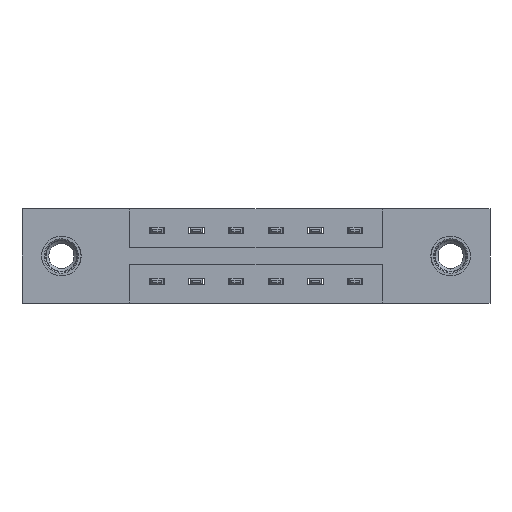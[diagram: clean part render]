
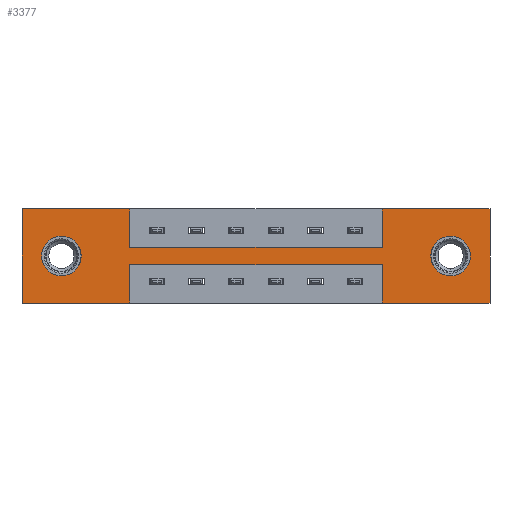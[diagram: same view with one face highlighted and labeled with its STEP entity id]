
A CAD part, front view. The second image highlights one B-rep face of the part: STEP entity #3377.
In plain terms, the highlighted planar face has unit normal (0, -1, 0).
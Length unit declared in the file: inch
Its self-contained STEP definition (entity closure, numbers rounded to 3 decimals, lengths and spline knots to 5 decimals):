
#58 = VECTOR ( 'NONE', #6489, 39.37008 ) ;
#78 = CARTESIAN_POINT ( 'NONE',  ( 0.425, 0., -0.22 ) ) ;
#393 = DIRECTION ( 'NONE',  ( 0., 1., 0. ) ) ;
#532 = DIRECTION ( 'NONE',  ( 0., 1., 0. ) ) ;
#810 = CARTESIAN_POINT ( 'NONE',  ( 0., 0., 0. ) ) ;
#1068 = DIRECTION ( 'NONE',  ( 0., 0., 1. ) ) ;
#1074 = DIRECTION ( 'NONE',  ( 0., 0., -1. ) ) ;
#1095 = CARTESIAN_POINT ( 'NONE',  ( 1.417, 0., -0.22 ) ) ;
#1121 = CARTESIAN_POINT ( 'NONE',  ( 1.687, 0., -0.263 ) ) ;
#1291 = ORIENTED_EDGE ( 'NONE', *, *, #8147, .F. ) ;
#1382 = ORIENTED_EDGE ( 'NONE', *, *, #4457, .F. ) ;
#1411 = EDGE_CURVE ( 'NONE', #7529, #3625, #1847, .T. ) ;
#1567 = EDGE_CURVE ( 'NONE', #8333, #8713, #4419, .T. ) ;
#1618 = DIRECTION ( 'NONE',  ( 0., 0., -1. ) ) ;
#1696 = EDGE_CURVE ( 'NONE', #7104, #2789, #3176, .T. ) ;
#1847 = LINE ( 'NONE', #6892, #4551 ) ;
#1904 = VECTOR ( 'NONE', #4253, 39.37008 ) ;
#2055 = CARTESIAN_POINT ( 'NONE',  ( 0.155, 0., -0.263 ) ) ;
#2165 = CARTESIAN_POINT ( 'NONE',  ( 1.842, 0., -0.37 ) ) ;
#2282 = CARTESIAN_POINT ( 'NONE',  ( 1.687, 0., -0.185 ) ) ;
#2416 = CARTESIAN_POINT ( 'NONE',  ( 0., 0., -0.37 ) ) ;
#2427 = LINE ( 'NONE', #2623, #8383 ) ;
#2592 = ORIENTED_EDGE ( 'NONE', *, *, #1411, .F. ) ;
#2623 = CARTESIAN_POINT ( 'NONE',  ( 1.842, 0., 0. ) ) ;
#2789 = VERTEX_POINT ( 'NONE', #9061 ) ;
#2800 = VERTEX_POINT ( 'NONE', #1121 ) ;
#2916 = DIRECTION ( 'NONE',  ( -1., 0., 0. ) ) ;
#3021 = EDGE_CURVE ( 'NONE', #3831, #3119, #7869, .T. ) ;
#3058 = AXIS2_PLACEMENT_3D ( 'NONE', #2416, #3770, #9369 ) ;
#3119 = VERTEX_POINT ( 'NONE', #6330 ) ;
#3174 = EDGE_CURVE ( 'NONE', #9122, #5603, #5626, .T. ) ;
#3176 = LINE ( 'NONE', #6428, #3908 ) ;
#3185 = AXIS2_PLACEMENT_3D ( 'NONE', #6871, #8557, #6077 ) ;
#3377 = ADVANCED_FACE ( 'NONE', ( #4749, #8250, #4385 ), #7163, .T. ) ;
#3480 = CARTESIAN_POINT ( 'NONE',  ( 1.417, 0., -0.37 ) ) ;
#3487 = CARTESIAN_POINT ( 'NONE',  ( 0.155, 0., -0.185 ) ) ;
#3557 = EDGE_CURVE ( 'NONE', #2800, #4116, #9262, .T. ) ;
#3574 = DIRECTION ( 'NONE',  ( 0., 0., 1. ) ) ;
#3625 = VERTEX_POINT ( 'NONE', #9545 ) ;
#3668 = DIRECTION ( 'NONE',  ( -1., 0., 0. ) ) ;
#3695 = CARTESIAN_POINT ( 'NONE',  ( 1.842, 0., 0. ) ) ;
#3770 = DIRECTION ( 'NONE',  ( 0., -1., 0. ) ) ;
#3831 = VERTEX_POINT ( 'NONE', #1095 ) ;
#3908 = VECTOR ( 'NONE', #9415, 39.37008 ) ;
#3991 = CARTESIAN_POINT ( 'NONE',  ( 0., 0., -0.37 ) ) ;
#4017 = CIRCLE ( 'NONE', #8345, 0.078 ) ;
#4115 = ORIENTED_EDGE ( 'NONE', *, *, #9272, .F. ) ;
#4116 = VERTEX_POINT ( 'NONE', #7068 ) ;
#4253 = DIRECTION ( 'NONE',  ( 1., 0., 0. ) ) ;
#4340 = LINE ( 'NONE', #9458, #9349 ) ;
#4358 = ORIENTED_EDGE ( 'NONE', *, *, #7783, .F. ) ;
#4385 = FACE_OUTER_BOUND ( 'NONE', #5245, .T. ) ;
#4419 = LINE ( 'NONE', #6917, #5160 ) ;
#4457 = EDGE_CURVE ( 'NONE', #6769, #7104, #4495, .T. ) ;
#4495 = LINE ( 'NONE', #5084, #1904 ) ;
#4551 = VECTOR ( 'NONE', #2916, 39.37008 ) ;
#4749 = FACE_BOUND ( 'NONE', #7474, .T. ) ;
#4874 = ORIENTED_EDGE ( 'NONE', *, *, #1696, .F. ) ;
#4905 = CARTESIAN_POINT ( 'NONE',  ( 0.425, 0., 0. ) ) ;
#4953 = ORIENTED_EDGE ( 'NONE', *, *, #7048, .F. ) ;
#4968 = CARTESIAN_POINT ( 'NONE',  ( 1.417, 0., -0.15 ) ) ;
#5084 = CARTESIAN_POINT ( 'NONE',  ( 0., 0., 0. ) ) ;
#5139 = ORIENTED_EDGE ( 'NONE', *, *, #9053, .T. ) ;
#5140 = ORIENTED_EDGE ( 'NONE', *, *, #3557, .T. ) ;
#5145 = LINE ( 'NONE', #810, #9289 ) ;
#5160 = VECTOR ( 'NONE', #5338, 39.37008 ) ;
#5245 = EDGE_LOOP ( 'NONE', ( #4953, #9064, #4358, #2592, #5509, #4115, #5807, #10116, #4874, #1382, #1291, #8521 ) ) ;
#5338 = DIRECTION ( 'NONE',  ( 0., 0., 1. ) ) ;
#5350 = EDGE_CURVE ( 'NONE', #2789, #8333, #4340, .T. ) ;
#5509 = ORIENTED_EDGE ( 'NONE', *, *, #9111, .F. ) ;
#5603 = VERTEX_POINT ( 'NONE', #6574 ) ;
#5626 = LINE ( 'NONE', #3991, #9633 ) ;
#5657 = CARTESIAN_POINT ( 'NONE',  ( 0., 0., 0. ) ) ;
#5807 = ORIENTED_EDGE ( 'NONE', *, *, #1567, .F. ) ;
#5898 = DIRECTION ( 'NONE',  ( 0., 0., 1. ) ) ;
#6077 = DIRECTION ( 'NONE',  ( 0., 0., -1. ) ) ;
#6239 = CARTESIAN_POINT ( 'NONE',  ( 0.425, 0., -0.37 ) ) ;
#6330 = CARTESIAN_POINT ( 'NONE',  ( 0.425, 0., -0.22 ) ) ;
#6336 = DIRECTION ( 'NONE',  ( 0., 0., 1. ) ) ;
#6371 = VECTOR ( 'NONE', #3668, 39.37008 ) ;
#6428 = CARTESIAN_POINT ( 'NONE',  ( 0.425, 0., 0. ) ) ;
#6489 = DIRECTION ( 'NONE',  ( 1., 0., 0. ) ) ;
#6550 = LINE ( 'NONE', #6862, #8673 ) ;
#6574 = CARTESIAN_POINT ( 'NONE',  ( 0., 0., -0.37 ) ) ;
#6769 = VERTEX_POINT ( 'NONE', #5657 ) ;
#6771 = LINE ( 'NONE', #3480, #8656 ) ;
#6862 = CARTESIAN_POINT ( 'NONE',  ( 0.425, 0., -0.37 ) ) ;
#6871 = CARTESIAN_POINT ( 'NONE',  ( 1.687, 0., -0.185 ) ) ;
#6892 = CARTESIAN_POINT ( 'NONE',  ( 0., 0., -0.37 ) ) ;
#6917 = CARTESIAN_POINT ( 'NONE',  ( 1.417, 0., 0. ) ) ;
#6945 = AXIS2_PLACEMENT_3D ( 'NONE', #3487, #393, #5898 ) ;
#7014 = VERTEX_POINT ( 'NONE', #2055 ) ;
#7048 = EDGE_CURVE ( 'NONE', #3119, #9122, #6550, .T. ) ;
#7068 = CARTESIAN_POINT ( 'NONE',  ( 1.687, 0., -0.107 ) ) ;
#7104 = VERTEX_POINT ( 'NONE', #4905 ) ;
#7163 = PLANE ( 'NONE',  #3058 ) ;
#7369 = CARTESIAN_POINT ( 'NONE',  ( 0., 0., 0. ) ) ;
#7474 = EDGE_LOOP ( 'NONE', ( #5139, #5140 ) ) ;
#7529 = VERTEX_POINT ( 'NONE', #2165 ) ;
#7636 = LINE ( 'NONE', #7369, #58 ) ;
#7638 = VERTEX_POINT ( 'NONE', #9795 ) ;
#7724 = DIRECTION ( 'NONE',  ( 1., 0., 0. ) ) ;
#7783 = EDGE_CURVE ( 'NONE', #3625, #3831, #6771, .T. ) ;
#7869 = LINE ( 'NONE', #78, #6371 ) ;
#8147 = EDGE_CURVE ( 'NONE', #5603, #6769, #5145, .T. ) ;
#8250 = FACE_BOUND ( 'NONE', #8601, .T. ) ;
#8333 = VERTEX_POINT ( 'NONE', #4968 ) ;
#8345 = AXIS2_PLACEMENT_3D ( 'NONE', #10039, #532, #3574 ) ;
#8383 = VECTOR ( 'NONE', #1074, 39.37008 ) ;
#8521 = ORIENTED_EDGE ( 'NONE', *, *, #3174, .F. ) ;
#8557 = DIRECTION ( 'NONE',  ( 0., 1., 0. ) ) ;
#8579 = ORIENTED_EDGE ( 'NONE', *, *, #8844, .T. ) ;
#8601 = EDGE_LOOP ( 'NONE', ( #9768, #8579 ) ) ;
#8647 = CIRCLE ( 'NONE', #9635, 0.078 ) ;
#8656 = VECTOR ( 'NONE', #1068, 39.37008 ) ;
#8673 = VECTOR ( 'NONE', #1618, 39.37008 ) ;
#8713 = VERTEX_POINT ( 'NONE', #9335 ) ;
#8844 = EDGE_CURVE ( 'NONE', #7014, #7638, #9661, .T. ) ;
#8969 = EDGE_CURVE ( 'NONE', #7638, #7014, #4017, .T. ) ;
#9053 = EDGE_CURVE ( 'NONE', #4116, #2800, #8647, .T. ) ;
#9061 = CARTESIAN_POINT ( 'NONE',  ( 0.425, 0., -0.15 ) ) ;
#9064 = ORIENTED_EDGE ( 'NONE', *, *, #3021, .F. ) ;
#9111 = EDGE_CURVE ( 'NONE', #9126, #7529, #2427, .T. ) ;
#9122 = VERTEX_POINT ( 'NONE', #6239 ) ;
#9126 = VERTEX_POINT ( 'NONE', #3695 ) ;
#9262 = CIRCLE ( 'NONE', #3185, 0.078 ) ;
#9272 = EDGE_CURVE ( 'NONE', #8713, #9126, #7636, .T. ) ;
#9289 = VECTOR ( 'NONE', #6336, 39.37008 ) ;
#9335 = CARTESIAN_POINT ( 'NONE',  ( 1.417, 0., 0. ) ) ;
#9349 = VECTOR ( 'NONE', #7724, 39.37008 ) ;
#9369 = DIRECTION ( 'NONE',  ( 0., 0., -1. ) ) ;
#9413 = DIRECTION ( 'NONE',  ( 0., 1., 0. ) ) ;
#9415 = DIRECTION ( 'NONE',  ( 0., 0., -1. ) ) ;
#9458 = CARTESIAN_POINT ( 'NONE',  ( 0.425, 0., -0.15 ) ) ;
#9545 = CARTESIAN_POINT ( 'NONE',  ( 1.417, 0., -0.37 ) ) ;
#9602 = DIRECTION ( 'NONE',  ( -1., 0., 0. ) ) ;
#9633 = VECTOR ( 'NONE', #9602, 39.37008 ) ;
#9635 = AXIS2_PLACEMENT_3D ( 'NONE', #2282, #9413, #10215 ) ;
#9661 = CIRCLE ( 'NONE', #6945, 0.078 ) ;
#9768 = ORIENTED_EDGE ( 'NONE', *, *, #8969, .T. ) ;
#9795 = CARTESIAN_POINT ( 'NONE',  ( 0.155, 0., -0.107 ) ) ;
#10039 = CARTESIAN_POINT ( 'NONE',  ( 0.155, 0., -0.185 ) ) ;
#10116 = ORIENTED_EDGE ( 'NONE', *, *, #5350, .F. ) ;
#10215 = DIRECTION ( 'NONE',  ( 0., 0., -1. ) ) ;
